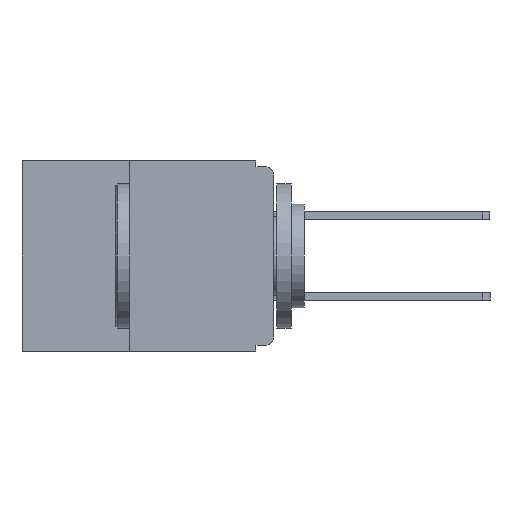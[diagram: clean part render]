
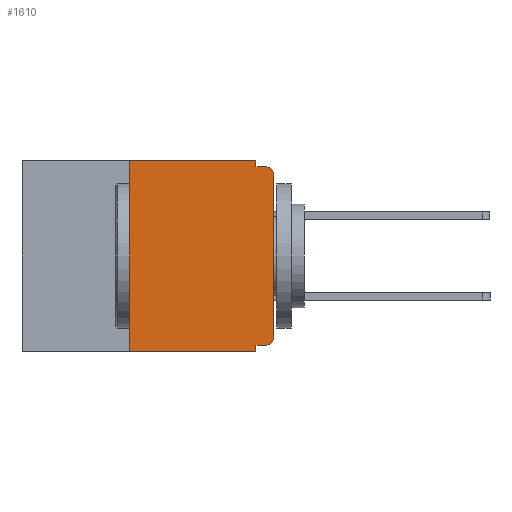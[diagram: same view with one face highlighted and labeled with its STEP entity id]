
A CAD part, left-side view. The second image highlights one B-rep face of the part: STEP entity #1610.
In plain terms, the highlighted planar face has unit normal (-1, 0, 0).
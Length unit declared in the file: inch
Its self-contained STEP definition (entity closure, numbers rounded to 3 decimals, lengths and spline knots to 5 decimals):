
#280 = ORIENTED_EDGE ( 'NONE', *, *, #3698, .F. ) ;
#291 = ORIENTED_EDGE ( 'NONE', *, *, #4526, .F. ) ;
#319 = CARTESIAN_POINT ( 'NONE',  ( 0., 0.437, 0. ) ) ;
#406 = CARTESIAN_POINT ( 'NONE',  ( 0., 0., -0.305 ) ) ;
#603 = LINE ( 'NONE', #9830, #12977 ) ;
#720 = EDGE_CURVE ( 'NONE', #3057, #3138, #11363, .T. ) ;
#780 = AXIS2_PLACEMENT_3D ( 'NONE', #7219, #10057, #9568 ) ;
#1105 = ORIENTED_EDGE ( 'NONE', *, *, #720, .T. ) ;
#1348 = VERTEX_POINT ( 'NONE', #7347 ) ;
#1396 = EDGE_LOOP ( 'NONE', ( #11307, #2808, #280, #291, #1963, #2443, #3163, #3437, #5086, #1105 ) ) ;
#1610 = ADVANCED_FACE ( 'NONE', ( #8999 ), #12096, .F. ) ;
#1627 = DIRECTION ( 'NONE',  ( 0., 0., 1. ) ) ;
#1637 = EDGE_CURVE ( 'NONE', #10713, #1348, #8948, .T. ) ;
#1850 = VERTEX_POINT ( 'NONE', #13088 ) ;
#1956 = DIRECTION ( 'NONE',  ( 0., 0., -1. ) ) ;
#1963 = ORIENTED_EDGE ( 'NONE', *, *, #11933, .F. ) ;
#1984 = DIRECTION ( 'NONE',  ( 0., 0., 1. ) ) ;
#2013 = VERTEX_POINT ( 'NONE', #10759 ) ;
#2062 = LINE ( 'NONE', #8932, #2094 ) ;
#2080 = CARTESIAN_POINT ( 'NONE',  ( 0., 0.031, -0.33 ) ) ;
#2094 = VECTOR ( 'NONE', #8804, 39.37008 ) ;
#2155 = CARTESIAN_POINT ( 'NONE',  ( 0., 0., 0. ) ) ;
#2443 = ORIENTED_EDGE ( 'NONE', *, *, #4019, .F. ) ;
#2577 = AXIS2_PLACEMENT_3D ( 'NONE', #7435, #8676, #8727 ) ;
#2714 = VERTEX_POINT ( 'NONE', #7859 ) ;
#2808 = ORIENTED_EDGE ( 'NONE', *, *, #1637, .T. ) ;
#2878 = AXIS2_PLACEMENT_3D ( 'NONE', #319, #12239, #12294 ) ;
#3057 = VERTEX_POINT ( 'NONE', #8602 ) ;
#3138 = VERTEX_POINT ( 'NONE', #406 ) ;
#3163 = ORIENTED_EDGE ( 'NONE', *, *, #3715, .T. ) ;
#3332 = VECTOR ( 'NONE', #1627, 39.37008 ) ;
#3393 = LINE ( 'NONE', #3482, #3332 ) ;
#3434 = VECTOR ( 'NONE', #1984, 39.37008 ) ;
#3437 = ORIENTED_EDGE ( 'NONE', *, *, #3440, .F. ) ;
#3440 = EDGE_CURVE ( 'NONE', #1850, #2013, #4797, .T. ) ;
#3461 = LINE ( 'NONE', #2155, #3434 ) ;
#3482 = CARTESIAN_POINT ( 'NONE',  ( 0., 0.25, -0.33 ) ) ;
#3698 = EDGE_CURVE ( 'NONE', #6170, #1348, #4326, .T. ) ;
#3715 = EDGE_CURVE ( 'NONE', #6164, #2013, #4182, .T. ) ;
#4019 = EDGE_CURVE ( 'NONE', #6164, #7827, #3393, .T. ) ;
#4182 = LINE ( 'NONE', #7508, #4258 ) ;
#4258 = VECTOR ( 'NONE', #7961, 39.37008 ) ;
#4326 = LINE ( 'NONE', #8337, #4338 ) ;
#4338 = VECTOR ( 'NONE', #8207, 39.37008 ) ;
#4526 = EDGE_CURVE ( 'NONE', #2714, #6170, #2062, .T. ) ;
#4695 = VECTOR ( 'NONE', #1956, 39.37008 ) ;
#4797 = LINE ( 'NONE', #2080, #4695 ) ;
#5086 = ORIENTED_EDGE ( 'NONE', *, *, #7596, .F. ) ;
#6164 = VERTEX_POINT ( 'NONE', #8340 ) ;
#6170 = VERTEX_POINT ( 'NONE', #8011 ) ;
#6577 = VECTOR ( 'NONE', #12171, 39.37008 ) ;
#6601 = LINE ( 'NONE', #10529, #6577 ) ;
#7041 = CARTESIAN_POINT ( 'NONE',  ( 0., 0., -0.025 ) ) ;
#7219 = CARTESIAN_POINT ( 'NONE',  ( 0., 0.015, -0.305 ) ) ;
#7347 = CARTESIAN_POINT ( 'NONE',  ( 0., 0.015, -0.01 ) ) ;
#7435 = CARTESIAN_POINT ( 'NONE',  ( 0., 0.015, -0.025 ) ) ;
#7508 = CARTESIAN_POINT ( 'NONE',  ( 0., 0.437, -0.33 ) ) ;
#7596 = EDGE_CURVE ( 'NONE', #3057, #1850, #6601, .T. ) ;
#7719 = CARTESIAN_POINT ( 'NONE',  ( 0., 0.25, 0. ) ) ;
#7827 = VERTEX_POINT ( 'NONE', #7719 ) ;
#7859 = CARTESIAN_POINT ( 'NONE',  ( 0., 0.031, 0. ) ) ;
#7961 = DIRECTION ( 'NONE',  ( 0., -1., 0. ) ) ;
#8011 = CARTESIAN_POINT ( 'NONE',  ( 0., 0.031, -0.01 ) ) ;
#8207 = DIRECTION ( 'NONE',  ( 0., -1., 0. ) ) ;
#8337 = CARTESIAN_POINT ( 'NONE',  ( 0., 0., -0.01 ) ) ;
#8340 = CARTESIAN_POINT ( 'NONE',  ( 0., 0.25, -0.33 ) ) ;
#8602 = CARTESIAN_POINT ( 'NONE',  ( 0., 0.015, -0.32 ) ) ;
#8676 = DIRECTION ( 'NONE',  ( -1., 0., 0. ) ) ;
#8727 = DIRECTION ( 'NONE',  ( 0., 0., -1. ) ) ;
#8804 = DIRECTION ( 'NONE',  ( 0., 0., -1. ) ) ;
#8932 = CARTESIAN_POINT ( 'NONE',  ( 0., 0.031, 0. ) ) ;
#8948 = CIRCLE ( 'NONE', #2577, 0.015 ) ;
#8999 = FACE_OUTER_BOUND ( 'NONE', #1396, .T. ) ;
#9568 = DIRECTION ( 'NONE',  ( 0., 0., -1. ) ) ;
#9797 = DIRECTION ( 'NONE',  ( 0., -1., 0. ) ) ;
#9830 = CARTESIAN_POINT ( 'NONE',  ( 0., 0.437, 0. ) ) ;
#10057 = DIRECTION ( 'NONE',  ( -1., 0., 0. ) ) ;
#10529 = CARTESIAN_POINT ( 'NONE',  ( 0., 0., -0.32 ) ) ;
#10713 = VERTEX_POINT ( 'NONE', #7041 ) ;
#10759 = CARTESIAN_POINT ( 'NONE',  ( 0., 0.031, -0.33 ) ) ;
#10866 = EDGE_CURVE ( 'NONE', #3138, #10713, #3461, .T. ) ;
#11307 = ORIENTED_EDGE ( 'NONE', *, *, #10866, .T. ) ;
#11363 = CIRCLE ( 'NONE', #780, 0.015 ) ;
#11933 = EDGE_CURVE ( 'NONE', #7827, #2714, #603, .T. ) ;
#12096 = PLANE ( 'NONE',  #2878 ) ;
#12171 = DIRECTION ( 'NONE',  ( 0., 1., 0. ) ) ;
#12239 = DIRECTION ( 'NONE',  ( 1., 0., 0. ) ) ;
#12294 = DIRECTION ( 'NONE',  ( 0., 0., -1. ) ) ;
#12977 = VECTOR ( 'NONE', #9797, 39.37008 ) ;
#13088 = CARTESIAN_POINT ( 'NONE',  ( 0., 0.031, -0.32 ) ) ;
